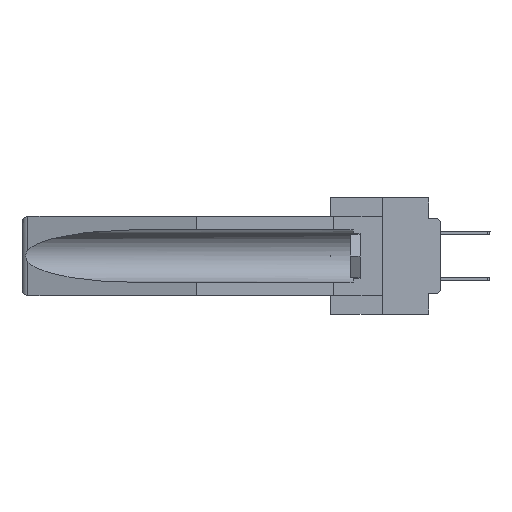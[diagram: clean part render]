
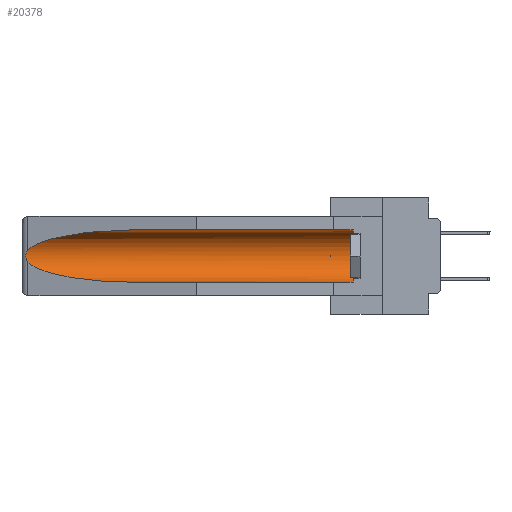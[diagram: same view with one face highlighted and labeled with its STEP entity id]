
A CAD part, left-side view. The second image highlights one B-rep face of the part: STEP entity #20378.
In plain terms, the highlighted cylindrical face has radius 2.857 mm (diameter 5.715 mm), a partial arc.
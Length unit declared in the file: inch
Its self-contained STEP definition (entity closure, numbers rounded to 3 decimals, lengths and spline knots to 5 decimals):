
#199 = CARTESIAN_POINT ( 'NONE',  ( 0.155, 1.07973, -0.059 ) ) ;
#262 = DIRECTION ( 'NONE',  ( 0., -1., 0. ) ) ;
#381 = CARTESIAN_POINT ( 'NONE',  ( 0.155, -0.30754, -0.1715 ) ) ;
#1695 = AXIS2_PLACEMENT_3D ( 'NONE', #18627, #262, #24811 ) ;
#2077 = EDGE_CURVE ( 'NONE', #36328, #16008, #37362, .T. ) ;
#2236 = CARTESIAN_POINT ( 'NONE',  ( 0.26655, 1.53094, -0.18657 ) ) ;
#3290 = ORIENTED_EDGE ( 'NONE', *, *, #16495, .T. ) ;
#4137 = ORIENTED_EDGE ( 'NONE', *, *, #2077, .F. ) ;
#4553 = ORIENTED_EDGE ( 'NONE', *, *, #22289, .T. ) ;
#5930 = CYLINDRICAL_SURFACE ( 'NONE', #32566, 0.1125 ) ;
#6492 = EDGE_CURVE ( 'NONE', #9731, #37898, #9278, .T. ) ;
#6672 = CARTESIAN_POINT ( 'NONE',  ( 0.26537, 1.52718, -0.14972 ) ) ;
#6786 = CARTESIAN_POINT ( 'NONE',  ( 0.26537, 1.52718, -0.19328 ) ) ;
#7639 = CARTESIAN_POINT ( 'NONE',  ( 0.155, 1.07973, -0.284 ) ) ;
#8264 = CARTESIAN_POINT ( 'NONE',  ( 0.2675, 1.53308, -0.16763 ) ) ;
#8408 = CARTESIAN_POINT ( 'NONE',  ( 0.26537, 1.52718, -0.14972 ) ) ;
#9278 = LINE ( 'NONE', #32931, #19794 ) ;
#9731 = VERTEX_POINT ( 'NONE', #34489 ) ;
#12335 = CARTESIAN_POINT ( 'NONE',  ( 0.25451, 1.48313, -0.09465 ) ) ;
#13381 = ORIENTED_EDGE ( 'NONE', *, *, #6492, .T. ) ;
#14076 = DIRECTION ( 'NONE',  ( 0., 1., 0. ) ) ;
#14184 = CARTESIAN_POINT ( 'NONE',  ( 0.2673, 1.5327, -0.16383 ) ) ;
#14495 = DIRECTION ( 'NONE',  ( 0., 1., 0. ) ) ;
#14594 = CARTESIAN_POINT ( 'NONE',  ( 0.26597, 1.5296, -0.19026 ) ) ;
#15132 =( BOUNDED_CURVE ( )  B_SPLINE_CURVE ( 3, ( #6786, #16061, #28540, #34887 ),
 .UNSPECIFIED., .F., .T. ) 
 B_SPLINE_CURVE_WITH_KNOTS ( ( 4, 4 ),
 ( 0.1948, 1.5708 ),
 .UNSPECIFIED. ) 
 CURVE ( )  GEOMETRIC_REPRESENTATION_ITEM ( )  RATIONAL_B_SPLINE_CURVE ( ( 1., 0.848, 0.848, 1. ) ) 
 REPRESENTATION_ITEM ( '' )  );
#15549 = CARTESIAN_POINT ( 'NONE',  ( 0.21114, 1.30732, -0.059 ) ) ;
#16008 = VERTEX_POINT ( 'NONE', #7639 ) ;
#16061 = CARTESIAN_POINT ( 'NONE',  ( 0.25451, 1.48313, -0.24835 ) ) ;
#16495 = EDGE_CURVE ( 'NONE', #37898, #34860, #20514, .T. ) ;
#17032 = FACE_OUTER_BOUND ( 'NONE', #34027, .T. ) ;
#17480 = ORIENTED_EDGE ( 'NONE', *, *, #18657, .T. ) ;
#17552 = CARTESIAN_POINT ( 'NONE',  ( 0.2675, 1.53308, -0.17534 ) ) ;
#18534 = EDGE_CURVE ( 'NONE', #38287, #16008, #15132, .T. ) ;
#18627 = CARTESIAN_POINT ( 'NONE',  ( 0.155, 0.126, -0.1715 ) ) ;
#18657 = EDGE_CURVE ( 'NONE', #34860, #38287, #23487, .T. ) ;
#19794 = VECTOR ( 'NONE', #14495, 39.37008 ) ;
#20378 = ADVANCED_FACE ( 'NONE', ( #17032 ), #5930, .F. ) ;
#20514 =( BOUNDED_CURVE ( )  B_SPLINE_CURVE ( 3, ( #25092, #15549, #12335, #6672 ),
 .UNSPECIFIED., .F., .F. ) 
 B_SPLINE_CURVE_WITH_KNOTS ( ( 4, 4 ),
 ( 4.71239, 6.08839 ),
 .UNSPECIFIED. ) 
 CURVE ( )  GEOMETRIC_REPRESENTATION_ITEM ( )  RATIONAL_B_SPLINE_CURVE ( ( 1., 0.848, 0.848, 1. ) ) 
 REPRESENTATION_ITEM ( '' )  );
#20635 = CARTESIAN_POINT ( 'NONE',  ( 0.155, -0.30754, -0.284 ) ) ;
#20738 = CARTESIAN_POINT ( 'NONE',  ( 0.26537, 1.52718, -0.19328 ) ) ;
#22289 = EDGE_CURVE ( 'NONE', #36328, #9731, #38403, .T. ) ;
#23487 = B_SPLINE_CURVE_WITH_KNOTS ( 'NONE', 3,
 ( #8408, #32629, #26670, #14184, #8264, #17552, #39059, #2236, #14594, #20738 ),
 .UNSPECIFIED., .F., .F.,
 ( 4, 2, 2, 2, 4 ),
 ( 0., 0.00029, 0.00058, 0.00087, 0.00117 ),
 .UNSPECIFIED. ) ;
#24353 = VECTOR ( 'NONE', #14076, 39.37008 ) ;
#24811 = DIRECTION ( 'NONE',  ( 0., 0., 1. ) ) ;
#25092 = CARTESIAN_POINT ( 'NONE',  ( 0.155, 1.07973, -0.059 ) ) ;
#26598 = CARTESIAN_POINT ( 'NONE',  ( 0.26537, 1.52718, -0.19328 ) ) ;
#26670 = CARTESIAN_POINT ( 'NONE',  ( 0.26654, 1.53092, -0.15636 ) ) ;
#28540 = CARTESIAN_POINT ( 'NONE',  ( 0.21114, 1.30732, -0.284 ) ) ;
#29874 = CARTESIAN_POINT ( 'NONE',  ( 0.155, 0.126, -0.284 ) ) ;
#32566 = AXIS2_PLACEMENT_3D ( 'NONE', #381, #37063, #37191 ) ;
#32629 = CARTESIAN_POINT ( 'NONE',  ( 0.26597, 1.52961, -0.15275 ) ) ;
#32931 = CARTESIAN_POINT ( 'NONE',  ( 0.155, -0.30754, -0.059 ) ) ;
#34027 = EDGE_LOOP ( 'NONE', ( #3290, #17480, #36464, #4137, #4553, #13381 ) ) ;
#34489 = CARTESIAN_POINT ( 'NONE',  ( 0.155, 0.126, -0.059 ) ) ;
#34860 = VERTEX_POINT ( 'NONE', #38321 ) ;
#34887 = CARTESIAN_POINT ( 'NONE',  ( 0.155, 1.07973, -0.284 ) ) ;
#36328 = VERTEX_POINT ( 'NONE', #29874 ) ;
#36464 = ORIENTED_EDGE ( 'NONE', *, *, #18534, .T. ) ;
#37063 = DIRECTION ( 'NONE',  ( 0., 1., 0. ) ) ;
#37191 = DIRECTION ( 'NONE',  ( 0., 0., 1. ) ) ;
#37362 = LINE ( 'NONE', #20635, #24353 ) ;
#37898 = VERTEX_POINT ( 'NONE', #199 ) ;
#38287 = VERTEX_POINT ( 'NONE', #26598 ) ;
#38321 = CARTESIAN_POINT ( 'NONE',  ( 0.26537, 1.52718, -0.14972 ) ) ;
#38403 = CIRCLE ( 'NONE', #1695, 0.1125 ) ;
#39059 = CARTESIAN_POINT ( 'NONE',  ( 0.2673, 1.53269, -0.17917 ) ) ;
